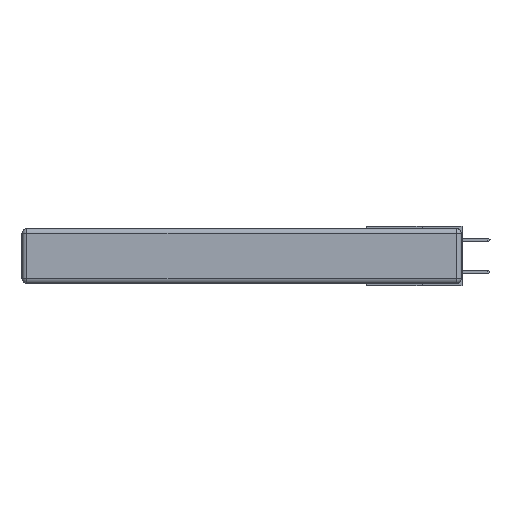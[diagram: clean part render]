
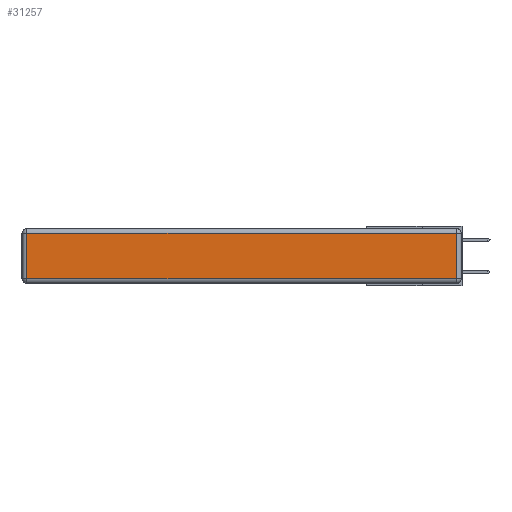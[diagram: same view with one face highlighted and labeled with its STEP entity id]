
A CAD part, left-side view. The second image highlights one B-rep face of the part: STEP entity #31257.
In plain terms, the highlighted planar face has unit normal (-1, 0, 0).
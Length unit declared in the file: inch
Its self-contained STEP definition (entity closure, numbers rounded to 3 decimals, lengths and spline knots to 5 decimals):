
#1029 = VERTEX_POINT ( 'NONE', #19911 ) ;
#2417 = VECTOR ( 'NONE', #23421, 39.37008 ) ;
#3385 = CARTESIAN_POINT ( 'NONE',  ( 0., 2.75, -0.03 ) ) ;
#3464 = VERTEX_POINT ( 'NONE', #31169 ) ;
#3527 = EDGE_CURVE ( 'NONE', #1029, #24229, #19511, .T. ) ;
#3592 = CARTESIAN_POINT ( 'NONE',  ( 0., 0.03, -0.03 ) ) ;
#3734 = FACE_OUTER_BOUND ( 'NONE', #9453, .T. ) ;
#5699 = CARTESIAN_POINT ( 'NONE',  ( 0., 0.03, -0.343 ) ) ;
#5849 = CARTESIAN_POINT ( 'NONE',  ( 0., 0., -0.343 ) ) ;
#5857 = DIRECTION ( 'NONE',  ( 0., 1., 0. ) ) ;
#8162 = CARTESIAN_POINT ( 'NONE',  ( 0., 0.03, -0.313 ) ) ;
#9453 = EDGE_LOOP ( 'NONE', ( #23945, #11622, #12737, #19279 ) ) ;
#10522 = VECTOR ( 'NONE', #23851, 39.37008 ) ;
#10981 = VECTOR ( 'NONE', #5857, 39.37008 ) ;
#11078 = LINE ( 'NONE', #15141, #11890 ) ;
#11350 = LINE ( 'NONE', #5699, #10522 ) ;
#11622 = ORIENTED_EDGE ( 'NONE', *, *, #14533, .T. ) ;
#11890 = VECTOR ( 'NONE', #12379, 39.37008 ) ;
#12379 = DIRECTION ( 'NONE',  ( 0., 0., -1. ) ) ;
#12737 = ORIENTED_EDGE ( 'NONE', *, *, #21023, .T. ) ;
#12970 = AXIS2_PLACEMENT_3D ( 'NONE', #5849, #31954, #16236 ) ;
#14032 = VERTEX_POINT ( 'NONE', #3592 ) ;
#14533 = EDGE_CURVE ( 'NONE', #24229, #14032, #11350, .T. ) ;
#15141 = CARTESIAN_POINT ( 'NONE',  ( 0., 2.72, -0.343 ) ) ;
#16236 = DIRECTION ( 'NONE',  ( 0., 0., 1. ) ) ;
#18595 = CARTESIAN_POINT ( 'NONE',  ( 0., 0., -0.313 ) ) ;
#18960 = PLANE ( 'NONE',  #12970 ) ;
#19279 = ORIENTED_EDGE ( 'NONE', *, *, #19548, .T. ) ;
#19511 = LINE ( 'NONE', #18595, #2417 ) ;
#19548 = EDGE_CURVE ( 'NONE', #3464, #1029, #11078, .T. ) ;
#19886 = LINE ( 'NONE', #3385, #10981 ) ;
#19911 = CARTESIAN_POINT ( 'NONE',  ( 0., 2.72, -0.313 ) ) ;
#21023 = EDGE_CURVE ( 'NONE', #14032, #3464, #19886, .T. ) ;
#23421 = DIRECTION ( 'NONE',  ( 0., -1., 0. ) ) ;
#23851 = DIRECTION ( 'NONE',  ( 0., 0., 1. ) ) ;
#23945 = ORIENTED_EDGE ( 'NONE', *, *, #3527, .T. ) ;
#24229 = VERTEX_POINT ( 'NONE', #8162 ) ;
#31169 = CARTESIAN_POINT ( 'NONE',  ( 0., 2.72, -0.03 ) ) ;
#31257 = ADVANCED_FACE ( 'NONE', ( #3734 ), #18960, .T. ) ;
#31954 = DIRECTION ( 'NONE',  ( -1., 0., 0. ) ) ;
